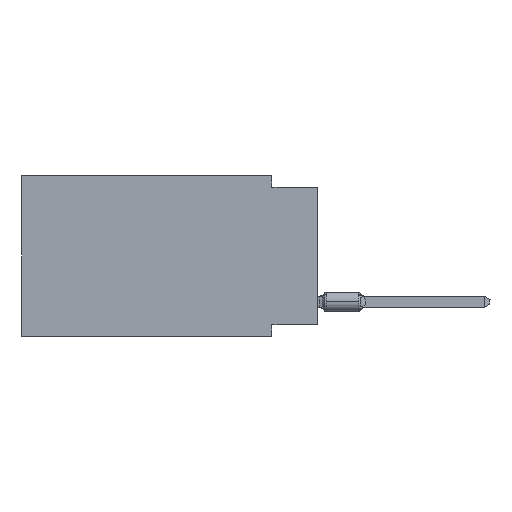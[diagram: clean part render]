
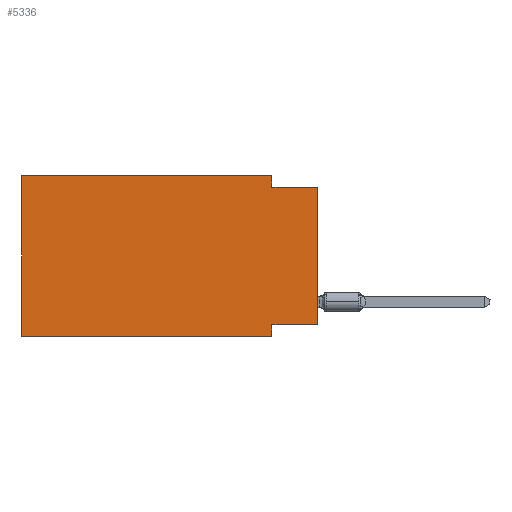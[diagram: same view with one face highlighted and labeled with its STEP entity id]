
A CAD part, left-side view. The second image highlights one B-rep face of the part: STEP entity #5336.
In plain terms, the highlighted planar face has unit normal (-1, 0, 0).
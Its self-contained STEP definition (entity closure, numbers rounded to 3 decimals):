
#2923 = DIRECTION ( 'NONE',  ( 0., 0., -1. ) ) ;
#4995 = CARTESIAN_POINT ( 'NONE',  ( 0., 2.54, -8.255 ) ) ;
#5176 = VECTOR ( 'NONE', #25275, 1000. ) ;
#5336 = ADVANCED_FACE ( 'NONE', ( #89057 ), #67770, .F. ) ;
#10514 = DIRECTION ( 'NONE',  ( 0., 0., 1. ) ) ;
#13270 = VERTEX_POINT ( 'NONE', #4995 ) ;
#15413 = VERTEX_POINT ( 'NONE', #18357 ) ;
#18357 = CARTESIAN_POINT ( 'NONE',  ( 0., 2.54, -8.89 ) ) ;
#19956 = CARTESIAN_POINT ( 'NONE',  ( 0., 16.383, -8.89 ) ) ;
#21169 = LINE ( 'NONE', #50045, #39896 ) ;
#22033 = CARTESIAN_POINT ( 'NONE',  ( 0., 0., -0.635 ) ) ;
#22255 = CARTESIAN_POINT ( 'NONE',  ( 0., 16.383, 0. ) ) ;
#22469 = CARTESIAN_POINT ( 'NONE',  ( 0., 2.54, -8.89 ) ) ;
#24745 = EDGE_CURVE ( 'NONE', #73819, #56890, #71261, .T. ) ;
#25258 = EDGE_CURVE ( 'NONE', #40069, #15413, #21169, .T. ) ;
#25275 = DIRECTION ( 'NONE',  ( 0., -1., 0. ) ) ;
#30148 = VECTOR ( 'NONE', #48141, 1000. ) ;
#31044 = CARTESIAN_POINT ( 'NONE',  ( 0., 2.54, -0.635 ) ) ;
#31046 = AXIS2_PLACEMENT_3D ( 'NONE', #45995, #81031, #2923 ) ;
#31149 = ORIENTED_EDGE ( 'NONE', *, *, #35957, .F. ) ;
#35393 = VERTEX_POINT ( 'NONE', #62975 ) ;
#35957 = EDGE_CURVE ( 'NONE', #13270, #15413, #87316, .T. ) ;
#39747 = ORIENTED_EDGE ( 'NONE', *, *, #25258, .T. ) ;
#39896 = VECTOR ( 'NONE', #78904, 1000. ) ;
#40069 = VERTEX_POINT ( 'NONE', #19956 ) ;
#41716 = CARTESIAN_POINT ( 'NONE',  ( 0., 16.383, 0. ) ) ;
#42002 = LINE ( 'NONE', #63776, #83475 ) ;
#42737 = VECTOR ( 'NONE', #51346, 1000. ) ;
#44479 = CARTESIAN_POINT ( 'NONE',  ( 0., 0., -8.255 ) ) ;
#45897 = VECTOR ( 'NONE', #57070, 1000. ) ;
#45995 = CARTESIAN_POINT ( 'NONE',  ( 0., 16.383, 0. ) ) ;
#46488 = LINE ( 'NONE', #75356, #68269 ) ;
#48141 = DIRECTION ( 'NONE',  ( 0., 0., -1. ) ) ;
#48303 = VERTEX_POINT ( 'NONE', #41716 ) ;
#49961 = EDGE_CURVE ( 'NONE', #84719, #56890, #89651, .T. ) ;
#50045 = CARTESIAN_POINT ( 'NONE',  ( 0., 16.383, -8.89 ) ) ;
#51346 = DIRECTION ( 'NONE',  ( 0., 0., -1. ) ) ;
#55265 = CARTESIAN_POINT ( 'NONE',  ( 0., 2.54, 0. ) ) ;
#56890 = VERTEX_POINT ( 'NONE', #22033 ) ;
#57042 = ORIENTED_EDGE ( 'NONE', *, *, #60748, .F. ) ;
#57070 = DIRECTION ( 'NONE',  ( 0., 0., 1. ) ) ;
#57101 = ORIENTED_EDGE ( 'NONE', *, *, #61719, .F. ) ;
#59896 = ORIENTED_EDGE ( 'NONE', *, *, #24745, .T. ) ;
#60748 = EDGE_CURVE ( 'NONE', #48303, #35393, #80001, .T. ) ;
#61719 = EDGE_CURVE ( 'NONE', #40069, #48303, #46488, .T. ) ;
#62792 = EDGE_LOOP ( 'NONE', ( #59896, #72227, #66894, #57042, #57101, #39747, #31149, #84707 ) ) ;
#62975 = CARTESIAN_POINT ( 'NONE',  ( 0., 2.54, 0. ) ) ;
#63776 = CARTESIAN_POINT ( 'NONE',  ( 0., 0., -8.255 ) ) ;
#64167 = CARTESIAN_POINT ( 'NONE',  ( 0., 0., 0. ) ) ;
#66894 = ORIENTED_EDGE ( 'NONE', *, *, #69802, .F. ) ;
#67770 = PLANE ( 'NONE',  #31046 ) ;
#68066 = LINE ( 'NONE', #55265, #30148 ) ;
#68136 = VECTOR ( 'NONE', #87563, 1000. ) ;
#68269 = VECTOR ( 'NONE', #10514, 1000. ) ;
#69802 = EDGE_CURVE ( 'NONE', #35393, #84719, #68066, .T. ) ;
#71261 = LINE ( 'NONE', #64167, #45897 ) ;
#72227 = ORIENTED_EDGE ( 'NONE', *, *, #49961, .F. ) ;
#73819 = VERTEX_POINT ( 'NONE', #44479 ) ;
#75356 = CARTESIAN_POINT ( 'NONE',  ( 0., 16.383, 0. ) ) ;
#78904 = DIRECTION ( 'NONE',  ( 0., -1., 0. ) ) ;
#78911 = DIRECTION ( 'NONE',  ( 0., 1., 0. ) ) ;
#80001 = LINE ( 'NONE', #22255, #68136 ) ;
#81031 = DIRECTION ( 'NONE',  ( 1., 0., 0. ) ) ;
#82547 = EDGE_CURVE ( 'NONE', #73819, #13270, #42002, .T. ) ;
#83475 = VECTOR ( 'NONE', #78911, 1000. ) ;
#84707 = ORIENTED_EDGE ( 'NONE', *, *, #82547, .F. ) ;
#84719 = VERTEX_POINT ( 'NONE', #31044 ) ;
#87316 = LINE ( 'NONE', #22469, #42737 ) ;
#87563 = DIRECTION ( 'NONE',  ( 0., -1., 0. ) ) ;
#88266 = CARTESIAN_POINT ( 'NONE',  ( 0., 0., -0.635 ) ) ;
#89057 = FACE_OUTER_BOUND ( 'NONE', #62792, .T. ) ;
#89651 = LINE ( 'NONE', #88266, #5176 ) ;
